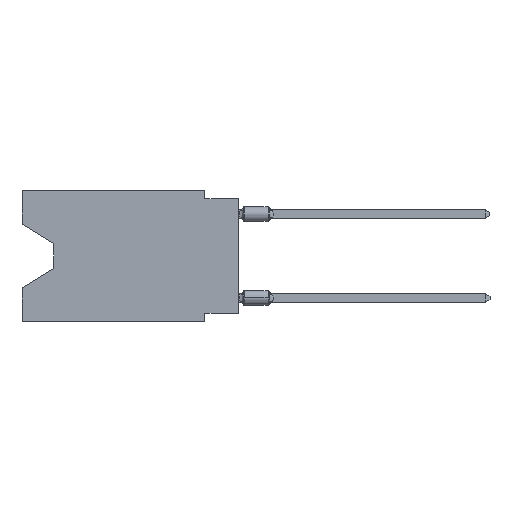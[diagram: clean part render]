
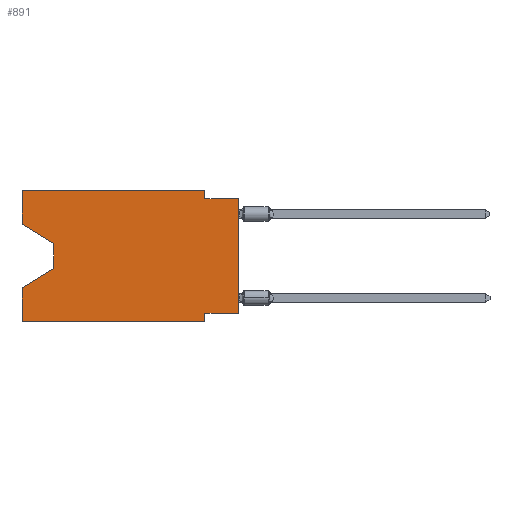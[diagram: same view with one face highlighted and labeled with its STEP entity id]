
A CAD part, left-side view. The second image highlights one B-rep face of the part: STEP entity #891.
In plain terms, the highlighted planar face has unit normal (-1, 0, 0).
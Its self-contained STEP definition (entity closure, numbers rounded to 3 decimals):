
#329 = EDGE_LOOP ( 'NONE', ( #23972, #19739, #11682, #1711, #14836, #3672, #11278, #16755, #15152, #13702, #2876, #20958 ) ) ;
#496 = VECTOR ( 'NONE', #2940, 1000. ) ;
#544 = CARTESIAN_POINT ( 'NONE',  ( 0., 16.383, -2.546 ) ) ;
#886 = VERTEX_POINT ( 'NONE', #22660 ) ;
#891 = ADVANCED_FACE ( 'NONE', ( #7744 ), #11040, .F. ) ;
#929 = EDGE_CURVE ( 'NONE', #23314, #3137, #9096, .T. ) ;
#979 = CARTESIAN_POINT ( 'NONE',  ( 0., 13.97, -4.013 ) ) ;
#1711 = ORIENTED_EDGE ( 'NONE', *, *, #19240, .F. ) ;
#2146 = EDGE_CURVE ( 'NONE', #7866, #886, #13124, .T. ) ;
#2744 = VECTOR ( 'NONE', #19946, 1000. ) ;
#2876 = ORIENTED_EDGE ( 'NONE', *, *, #4068, .F. ) ;
#2940 = DIRECTION ( 'NONE',  ( 0., 0., -1. ) ) ;
#3137 = VERTEX_POINT ( 'NONE', #22312 ) ;
#3343 = VERTEX_POINT ( 'NONE', #16533 ) ;
#3363 = CARTESIAN_POINT ( 'NONE',  ( 0., 16.383, -9.906 ) ) ;
#3672 = ORIENTED_EDGE ( 'NONE', *, *, #23688, .F. ) ;
#3810 = CARTESIAN_POINT ( 'NONE',  ( 0., 2.54, 0. ) ) ;
#3963 = VECTOR ( 'NONE', #4616, 1000. ) ;
#4067 = DIRECTION ( 'NONE',  ( 0., 0., -1. ) ) ;
#4068 = EDGE_CURVE ( 'NONE', #5990, #7866, #21396, .T. ) ;
#4481 = VECTOR ( 'NONE', #22172, 1000. ) ;
#4616 = DIRECTION ( 'NONE',  ( 0., -1., 0. ) ) ;
#4797 = EDGE_CURVE ( 'NONE', #3137, #3343, #8342, .T. ) ;
#5059 = DIRECTION ( 'NONE',  ( 0., 0., 1. ) ) ;
#5990 = VERTEX_POINT ( 'NONE', #8827 ) ;
#6385 = CARTESIAN_POINT ( 'NONE',  ( 0., 0., -0.635 ) ) ;
#6693 = DIRECTION ( 'NONE',  ( 0., -1., 0. ) ) ;
#6865 = LINE ( 'NONE', #21794, #2744 ) ;
#7299 = VECTOR ( 'NONE', #21773, 1000. ) ;
#7744 = FACE_OUTER_BOUND ( 'NONE', #329, .T. ) ;
#7866 = VERTEX_POINT ( 'NONE', #17675 ) ;
#8342 = LINE ( 'NONE', #979, #496 ) ;
#8827 = CARTESIAN_POINT ( 'NONE',  ( 0., 16.383, 0. ) ) ;
#9029 = CARTESIAN_POINT ( 'NONE',  ( 0., 16.383, 0. ) ) ;
#9096 = LINE ( 'NONE', #23998, #4481 ) ;
#9346 = VERTEX_POINT ( 'NONE', #11770 ) ;
#10703 = VECTOR ( 'NONE', #5059, 1000. ) ;
#11040 = PLANE ( 'NONE',  #14620 ) ;
#11271 = EDGE_CURVE ( 'NONE', #9346, #13473, #6865, .T. ) ;
#11278 = ORIENTED_EDGE ( 'NONE', *, *, #14243, .F. ) ;
#11291 = VERTEX_POINT ( 'NONE', #16399 ) ;
#11294 = DIRECTION ( 'NONE',  ( 0., 0., -1. ) ) ;
#11682 = ORIENTED_EDGE ( 'NONE', *, *, #12463, .T. ) ;
#11770 = CARTESIAN_POINT ( 'NONE',  ( 0., 0., -9.271 ) ) ;
#12378 = VERTEX_POINT ( 'NONE', #15688 ) ;
#12463 = EDGE_CURVE ( 'NONE', #3343, #12378, #23734, .T. ) ;
#12563 = LINE ( 'NONE', #3363, #24054 ) ;
#13124 = LINE ( 'NONE', #3810, #21179 ) ;
#13473 = VERTEX_POINT ( 'NONE', #15991 ) ;
#13478 = EDGE_CURVE ( 'NONE', #14899, #14587, #12563, .T. ) ;
#13702 = ORIENTED_EDGE ( 'NONE', *, *, #2146, .F. ) ;
#13918 = CARTESIAN_POINT ( 'NONE',  ( 0., 2.54, -9.906 ) ) ;
#14243 = EDGE_CURVE ( 'NONE', #9346, #11291, #16139, .T. ) ;
#14587 = VERTEX_POINT ( 'NONE', #13918 ) ;
#14620 = AXIS2_PLACEMENT_3D ( 'NONE', #18489, #15060, #18615 ) ;
#14671 = DIRECTION ( 'NONE',  ( 0., 0.855, -0.519 ) ) ;
#14825 = VECTOR ( 'NONE', #19585, 1000. ) ;
#14836 = ORIENTED_EDGE ( 'NONE', *, *, #13478, .T. ) ;
#14899 = VERTEX_POINT ( 'NONE', #22337 ) ;
#15060 = DIRECTION ( 'NONE',  ( 1., 0., 0. ) ) ;
#15152 = ORIENTED_EDGE ( 'NONE', *, *, #17251, .F. ) ;
#15198 = CARTESIAN_POINT ( 'NONE',  ( 0., 2.54, -9.906 ) ) ;
#15682 = LINE ( 'NONE', #6385, #14825 ) ;
#15688 = CARTESIAN_POINT ( 'NONE',  ( 0., 16.383, -7.36 ) ) ;
#15991 = CARTESIAN_POINT ( 'NONE',  ( 0., 0., -0.635 ) ) ;
#16139 = LINE ( 'NONE', #22121, #7299 ) ;
#16399 = CARTESIAN_POINT ( 'NONE',  ( 0., 2.54, -9.271 ) ) ;
#16533 = CARTESIAN_POINT ( 'NONE',  ( 0., 13.97, -5.893 ) ) ;
#16728 = LINE ( 'NONE', #9029, #23959 ) ;
#16755 = ORIENTED_EDGE ( 'NONE', *, *, #11271, .T. ) ;
#17251 = EDGE_CURVE ( 'NONE', #886, #13473, #15682, .T. ) ;
#17675 = CARTESIAN_POINT ( 'NONE',  ( 0., 2.54, 0. ) ) ;
#18489 = CARTESIAN_POINT ( 'NONE',  ( 0., 16.383, 0. ) ) ;
#18615 = DIRECTION ( 'NONE',  ( 0., 0., -1. ) ) ;
#18939 = VECTOR ( 'NONE', #14671, 1000. ) ;
#18956 = EDGE_CURVE ( 'NONE', #23314, #5990, #16728, .T. ) ;
#19240 = EDGE_CURVE ( 'NONE', #14899, #12378, #23427, .T. ) ;
#19585 = DIRECTION ( 'NONE',  ( 0., -1., 0. ) ) ;
#19725 = VECTOR ( 'NONE', #4067, 1000. ) ;
#19739 = ORIENTED_EDGE ( 'NONE', *, *, #4797, .T. ) ;
#19946 = DIRECTION ( 'NONE',  ( 0., 0., 1. ) ) ;
#20958 = ORIENTED_EDGE ( 'NONE', *, *, #18956, .F. ) ;
#21179 = VECTOR ( 'NONE', #11294, 1000. ) ;
#21396 = LINE ( 'NONE', #21511, #3963 ) ;
#21488 = CARTESIAN_POINT ( 'NONE',  ( 0., 16.383, 0. ) ) ;
#21511 = CARTESIAN_POINT ( 'NONE',  ( 0., 16.383, 0. ) ) ;
#21773 = DIRECTION ( 'NONE',  ( 0., 1., 0. ) ) ;
#21794 = CARTESIAN_POINT ( 'NONE',  ( 0., 0., 0. ) ) ;
#21800 = CARTESIAN_POINT ( 'NONE',  ( 0., 13.97, -5.893 ) ) ;
#22121 = CARTESIAN_POINT ( 'NONE',  ( 0., 0., -9.271 ) ) ;
#22172 = DIRECTION ( 'NONE',  ( 0., -0.855, -0.519 ) ) ;
#22312 = CARTESIAN_POINT ( 'NONE',  ( 0., 13.97, -4.013 ) ) ;
#22337 = CARTESIAN_POINT ( 'NONE',  ( 0., 16.383, -9.906 ) ) ;
#22421 = LINE ( 'NONE', #15198, #19725 ) ;
#22660 = CARTESIAN_POINT ( 'NONE',  ( 0., 2.54, -0.635 ) ) ;
#23314 = VERTEX_POINT ( 'NONE', #544 ) ;
#23427 = LINE ( 'NONE', #21488, #10703 ) ;
#23688 = EDGE_CURVE ( 'NONE', #11291, #14587, #22421, .T. ) ;
#23734 = LINE ( 'NONE', #21800, #18939 ) ;
#23959 = VECTOR ( 'NONE', #24161, 1000. ) ;
#23972 = ORIENTED_EDGE ( 'NONE', *, *, #929, .T. ) ;
#23998 = CARTESIAN_POINT ( 'NONE',  ( 0., 16.383, -2.546 ) ) ;
#24054 = VECTOR ( 'NONE', #6693, 1000. ) ;
#24161 = DIRECTION ( 'NONE',  ( 0., 0., 1. ) ) ;
